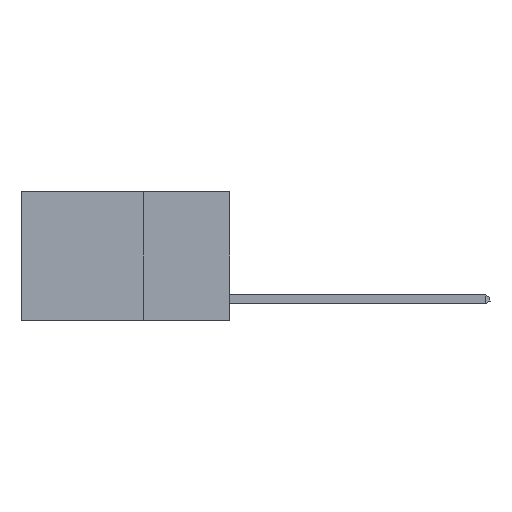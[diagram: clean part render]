
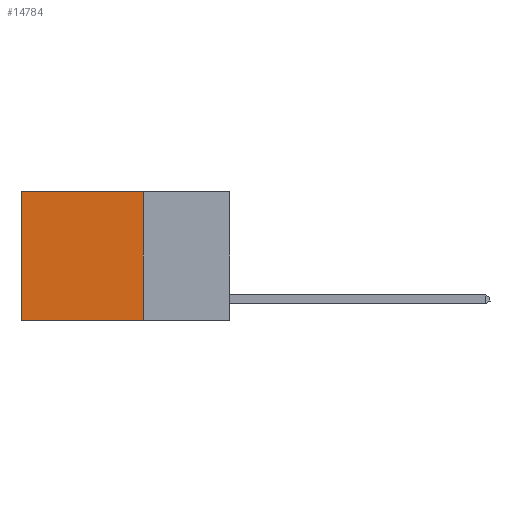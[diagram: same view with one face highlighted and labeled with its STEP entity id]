
A CAD part, left-side view. The second image highlights one B-rep face of the part: STEP entity #14784.
In plain terms, the highlighted planar face has unit normal (-1, 0, 0).
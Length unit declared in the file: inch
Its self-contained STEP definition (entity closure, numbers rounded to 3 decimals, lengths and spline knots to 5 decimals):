
#1747 = VERTEX_POINT ( 'NONE', #22210 ) ;
#1936 = VECTOR ( 'NONE', #5138, 39.37008 ) ;
#2789 = CARTESIAN_POINT ( 'NONE',  ( 0.2625, 0.6, 0. ) ) ;
#3993 = LINE ( 'NONE', #23225, #10172 ) ;
#4304 = DIRECTION ( 'NONE',  ( 1., 0., 0. ) ) ;
#4861 = EDGE_CURVE ( 'NONE', #5058, #24334, #12704, .T. ) ;
#5058 = VERTEX_POINT ( 'NONE', #27588 ) ;
#5132 = FACE_OUTER_BOUND ( 'NONE', #23830, .T. ) ;
#5138 = DIRECTION ( 'NONE',  ( 0., 0., -1. ) ) ;
#5676 = EDGE_CURVE ( 'NONE', #11647, #5058, #3993, .T. ) ;
#5836 = DIRECTION ( 'NONE',  ( 0., 1., 0. ) ) ;
#6571 = ORIENTED_EDGE ( 'NONE', *, *, #15688, .T. ) ;
#7112 = ORIENTED_EDGE ( 'NONE', *, *, #19924, .T. ) ;
#8813 = LINE ( 'NONE', #2789, #1936 ) ;
#10172 = VECTOR ( 'NONE', #25485, 39.37008 ) ;
#10896 = VECTOR ( 'NONE', #5836, 39.37008 ) ;
#11117 = CARTESIAN_POINT ( 'NONE',  ( 0.2625, 0.25, 0. ) ) ;
#11647 = VERTEX_POINT ( 'NONE', #11117 ) ;
#12016 = ORIENTED_EDGE ( 'NONE', *, *, #4861, .F. ) ;
#12704 = LINE ( 'NONE', #17539, #18049 ) ;
#12961 = DIRECTION ( 'NONE',  ( 0., 1., 0. ) ) ;
#14721 = AXIS2_PLACEMENT_3D ( 'NONE', #18056, #4304, #20341 ) ;
#14784 = ADVANCED_FACE ( 'NONE', ( #5132 ), #29249, .F. ) ;
#15688 = EDGE_CURVE ( 'NONE', #11647, #1747, #16219, .T. ) ;
#16219 = LINE ( 'NONE', #19557, #10896 ) ;
#16823 = CARTESIAN_POINT ( 'NONE',  ( 0.2625, 0.6, -0.37 ) ) ;
#17539 = CARTESIAN_POINT ( 'NONE',  ( 0.2625, 0.25, -0.37 ) ) ;
#18049 = VECTOR ( 'NONE', #12961, 39.37008 ) ;
#18056 = CARTESIAN_POINT ( 'NONE',  ( 0.2625, 0.25, 0. ) ) ;
#18948 = ORIENTED_EDGE ( 'NONE', *, *, #5676, .F. ) ;
#19557 = CARTESIAN_POINT ( 'NONE',  ( 0.2625, 0.25, 0. ) ) ;
#19924 = EDGE_CURVE ( 'NONE', #1747, #24334, #8813, .T. ) ;
#20341 = DIRECTION ( 'NONE',  ( 0., 0., -1. ) ) ;
#22210 = CARTESIAN_POINT ( 'NONE',  ( 0.2625, 0.6, 0. ) ) ;
#23225 = CARTESIAN_POINT ( 'NONE',  ( 0.2625, 0.25, 0. ) ) ;
#23830 = EDGE_LOOP ( 'NONE', ( #7112, #12016, #18948, #6571 ) ) ;
#24334 = VERTEX_POINT ( 'NONE', #16823 ) ;
#25485 = DIRECTION ( 'NONE',  ( 0., 0., -1. ) ) ;
#27588 = CARTESIAN_POINT ( 'NONE',  ( 0.2625, 0.25, -0.37 ) ) ;
#29249 = PLANE ( 'NONE',  #14721 ) ;
